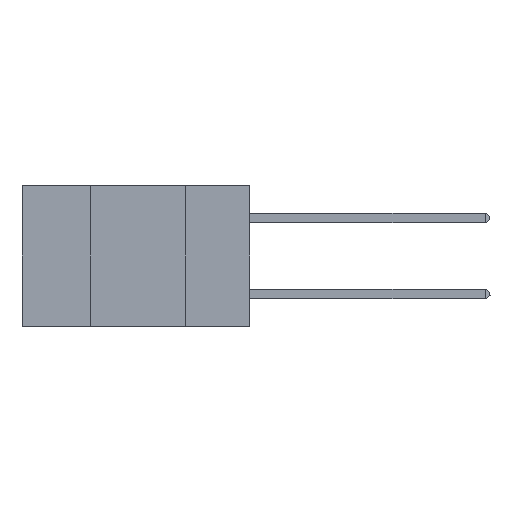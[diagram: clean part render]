
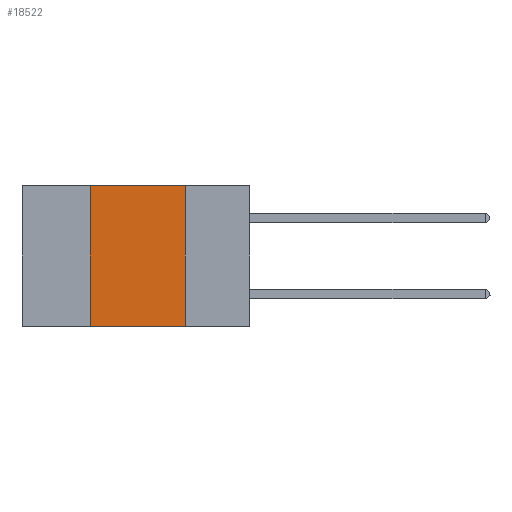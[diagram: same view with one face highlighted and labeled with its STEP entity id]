
A CAD part, left-side view. The second image highlights one B-rep face of the part: STEP entity #18522.
In plain terms, the highlighted planar face has unit normal (-1, 0, 0).
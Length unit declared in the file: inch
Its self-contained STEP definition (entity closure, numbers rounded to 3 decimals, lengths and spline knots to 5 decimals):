
#187 = DIRECTION ( 'NONE',  ( 0., 0., -1. ) ) ;
#304 = LINE ( 'NONE', #28024, #8404 ) ;
#516 = VERTEX_POINT ( 'NONE', #20600 ) ;
#810 = LINE ( 'NONE', #25845, #19197 ) ;
#903 = CARTESIAN_POINT ( 'NONE',  ( 0., 0.17, 0. ) ) ;
#1301 = CARTESIAN_POINT ( 'NONE',  ( 0., 0.42, 0. ) ) ;
#1750 = LINE ( 'NONE', #6615, #13098 ) ;
#2109 = DIRECTION ( 'NONE',  ( 0., -1., 0. ) ) ;
#3122 = VERTEX_POINT ( 'NONE', #903 ) ;
#3988 = FACE_OUTER_BOUND ( 'NONE', #22145, .T. ) ;
#4487 = ORIENTED_EDGE ( 'NONE', *, *, #19738, .F. ) ;
#6208 = DIRECTION ( 'NONE',  ( 0., 0., -1. ) ) ;
#6615 = CARTESIAN_POINT ( 'NONE',  ( 0., 0.6, 0. ) ) ;
#8404 = VECTOR ( 'NONE', #30392, 39.37008 ) ;
#10659 = ORIENTED_EDGE ( 'NONE', *, *, #23589, .F. ) ;
#11277 = EDGE_CURVE ( 'NONE', #24458, #516, #304, .T. ) ;
#11631 = ORIENTED_EDGE ( 'NONE', *, *, #11277, .T. ) ;
#11750 = LINE ( 'NONE', #23707, #26106 ) ;
#13098 = VECTOR ( 'NONE', #2109, 39.37008 ) ;
#18094 = EDGE_CURVE ( 'NONE', #3122, #516, #11750, .T. ) ;
#18522 = ADVANCED_FACE ( 'NONE', ( #3988 ), #27674, .F. ) ;
#19197 = VECTOR ( 'NONE', #23402, 39.37008 ) ;
#19738 = EDGE_CURVE ( 'NONE', #25680, #3122, #1750, .T. ) ;
#20526 = CARTESIAN_POINT ( 'NONE',  ( 0., 0.6, 0. ) ) ;
#20600 = CARTESIAN_POINT ( 'NONE',  ( 0., 0.17, -0.37 ) ) ;
#22145 = EDGE_LOOP ( 'NONE', ( #22344, #4487, #10659, #11631 ) ) ;
#22344 = ORIENTED_EDGE ( 'NONE', *, *, #18094, .F. ) ;
#22652 = DIRECTION ( 'NONE',  ( 1., 0., 0. ) ) ;
#23402 = DIRECTION ( 'NONE',  ( 0., 0., 1. ) ) ;
#23589 = EDGE_CURVE ( 'NONE', #24458, #25680, #810, .T. ) ;
#23707 = CARTESIAN_POINT ( 'NONE',  ( 0., 0.17, 0. ) ) ;
#24458 = VERTEX_POINT ( 'NONE', #26703 ) ;
#25680 = VERTEX_POINT ( 'NONE', #1301 ) ;
#25845 = CARTESIAN_POINT ( 'NONE',  ( 0., 0.42, 0. ) ) ;
#25980 = AXIS2_PLACEMENT_3D ( 'NONE', #20526, #22652, #6208 ) ;
#26106 = VECTOR ( 'NONE', #187, 39.37008 ) ;
#26703 = CARTESIAN_POINT ( 'NONE',  ( 0., 0.42, -0.37 ) ) ;
#27674 = PLANE ( 'NONE',  #25980 ) ;
#28024 = CARTESIAN_POINT ( 'NONE',  ( 0., 0.6, -0.37 ) ) ;
#30392 = DIRECTION ( 'NONE',  ( 0., -1., 0. ) ) ;
